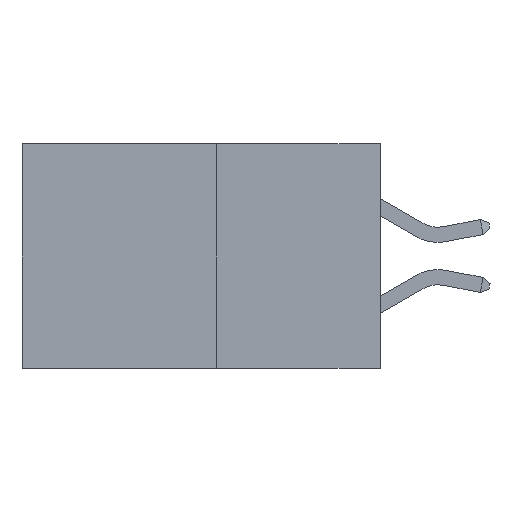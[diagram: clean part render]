
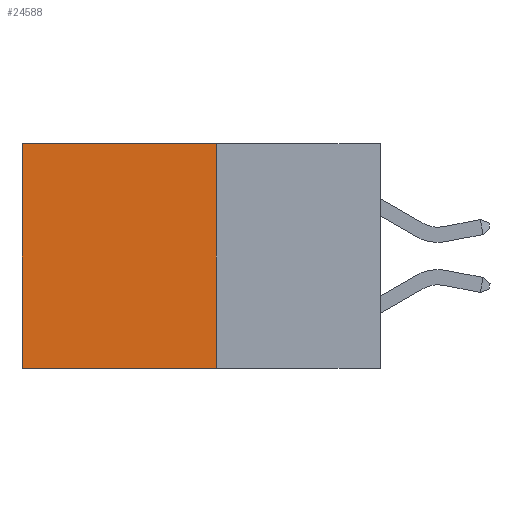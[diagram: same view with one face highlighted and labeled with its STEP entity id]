
A CAD part, left-side view. The second image highlights one B-rep face of the part: STEP entity #24588.
In plain terms, the highlighted planar face has unit normal (-1, 0, 0).
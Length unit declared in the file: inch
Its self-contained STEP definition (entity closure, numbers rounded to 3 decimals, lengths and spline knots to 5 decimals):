
#298 = LINE ( 'NONE', #9237, #17803 ) ;
#1542 = VECTOR ( 'NONE', #12823, 39.37008 ) ;
#1709 = ORIENTED_EDGE ( 'NONE', *, *, #20858, .T. ) ;
#1962 = CARTESIAN_POINT ( 'NONE',  ( 0.277, 0.27, 0. ) ) ;
#2233 = ORIENTED_EDGE ( 'NONE', *, *, #25300, .T. ) ;
#2358 = VECTOR ( 'NONE', #6881, 39.37008 ) ;
#3085 = DIRECTION ( 'NONE',  ( 0., 0., -1. ) ) ;
#3098 = VERTEX_POINT ( 'NONE', #19922 ) ;
#3497 = CARTESIAN_POINT ( 'NONE',  ( 0.277, 0.27, -0.37 ) ) ;
#4157 = ORIENTED_EDGE ( 'NONE', *, *, #17378, .F. ) ;
#4666 = CARTESIAN_POINT ( 'NONE',  ( 0.277, 0.27, -0.37 ) ) ;
#5713 = DIRECTION ( 'NONE',  ( 0., 0., -1. ) ) ;
#6881 = DIRECTION ( 'NONE',  ( 0., 1., 0. ) ) ;
#9237 = CARTESIAN_POINT ( 'NONE',  ( 0.277, 0.59, -0.37 ) ) ;
#9660 = CARTESIAN_POINT ( 'NONE',  ( 0.277, 0.27, -0.37 ) ) ;
#10708 = EDGE_LOOP ( 'NONE', ( #1709, #11287, #4157, #2233 ) ) ;
#11287 = ORIENTED_EDGE ( 'NONE', *, *, #20813, .F. ) ;
#12095 = FACE_OUTER_BOUND ( 'NONE', #10708, .T. ) ;
#12823 = DIRECTION ( 'NONE',  ( 0., 1., 0. ) ) ;
#14355 = AXIS2_PLACEMENT_3D ( 'NONE', #3497, #18872, #5713 ) ;
#14405 = VECTOR ( 'NONE', #3085, 39.37008 ) ;
#14548 = VERTEX_POINT ( 'NONE', #18290 ) ;
#14908 = VERTEX_POINT ( 'NONE', #1962 ) ;
#16622 = PLANE ( 'NONE',  #14355 ) ;
#17378 = EDGE_CURVE ( 'NONE', #14908, #20745, #25897, .T. ) ;
#17803 = VECTOR ( 'NONE', #20095, 39.37008 ) ;
#18290 = CARTESIAN_POINT ( 'NONE',  ( 0.277, 0.59, 0. ) ) ;
#18872 = DIRECTION ( 'NONE',  ( 1., 0., 0. ) ) ;
#19922 = CARTESIAN_POINT ( 'NONE',  ( 0.277, 0.59, -0.37 ) ) ;
#20095 = DIRECTION ( 'NONE',  ( 0., 0., -1. ) ) ;
#20745 = VERTEX_POINT ( 'NONE', #26267 ) ;
#20813 = EDGE_CURVE ( 'NONE', #20745, #3098, #24195, .T. ) ;
#20858 = EDGE_CURVE ( 'NONE', #14548, #3098, #298, .T. ) ;
#21466 = CARTESIAN_POINT ( 'NONE',  ( 0.277, 0.27, 0. ) ) ;
#23244 = LINE ( 'NONE', #21466, #1542 ) ;
#24195 = LINE ( 'NONE', #4666, #2358 ) ;
#24588 = ADVANCED_FACE ( 'NONE', ( #12095 ), #16622, .F. ) ;
#25300 = EDGE_CURVE ( 'NONE', #14908, #14548, #23244, .T. ) ;
#25897 = LINE ( 'NONE', #9660, #14405 ) ;
#26267 = CARTESIAN_POINT ( 'NONE',  ( 0.277, 0.27, -0.37 ) ) ;
